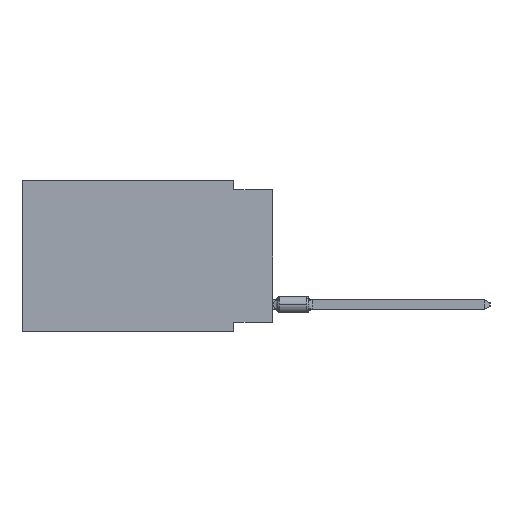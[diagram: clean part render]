
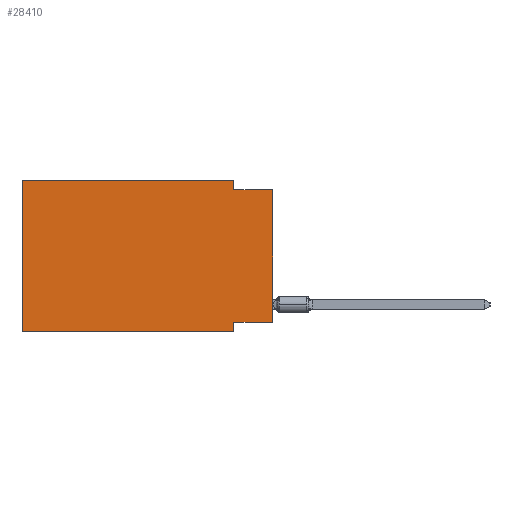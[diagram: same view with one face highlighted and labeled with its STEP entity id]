
A CAD part, left-side view. The second image highlights one B-rep face of the part: STEP entity #28410.
In plain terms, the highlighted planar face has unit normal (-1, 0, 0).
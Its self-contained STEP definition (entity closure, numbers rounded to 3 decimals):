
#1242 = DIRECTION ( 'NONE',  ( 0., 0., -1. ) ) ;
#1474 = CARTESIAN_POINT ( 'NONE',  ( 0., 0., -9.271 ) ) ;
#2126 = PLANE ( 'NONE',  #21336 ) ;
#3246 = VERTEX_POINT ( 'NONE', #35363 ) ;
#3310 = VERTEX_POINT ( 'NONE', #5053 ) ;
#4761 = CARTESIAN_POINT ( 'NONE',  ( 0., 2.54, -0.635 ) ) ;
#5053 = CARTESIAN_POINT ( 'NONE',  ( 0., 2.54, -9.906 ) ) ;
#6661 = ORIENTED_EDGE ( 'NONE', *, *, #19659, .F. ) ;
#7812 = VECTOR ( 'NONE', #42148, 1000. ) ;
#8633 = LINE ( 'NONE', #20342, #9895 ) ;
#8875 = CARTESIAN_POINT ( 'NONE',  ( 0., 16.383, 0. ) ) ;
#9584 = DIRECTION ( 'NONE',  ( 1., 0., 0. ) ) ;
#9895 = VECTOR ( 'NONE', #32807, 1000. ) ;
#10799 = CARTESIAN_POINT ( 'NONE',  ( 0., 0., 0. ) ) ;
#10932 = VECTOR ( 'NONE', #20970, 1000. ) ;
#11849 = DIRECTION ( 'NONE',  ( 0., -1., 0. ) ) ;
#11919 = CARTESIAN_POINT ( 'NONE',  ( 0., 16.383, 0. ) ) ;
#14776 = VERTEX_POINT ( 'NONE', #19033 ) ;
#14794 = LINE ( 'NONE', #25578, #43754 ) ;
#15599 = LINE ( 'NONE', #31794, #17666 ) ;
#17247 = VERTEX_POINT ( 'NONE', #35749 ) ;
#17666 = VECTOR ( 'NONE', #11849, 1000. ) ;
#18080 = VERTEX_POINT ( 'NONE', #1474 ) ;
#19033 = CARTESIAN_POINT ( 'NONE',  ( 0., 2.54, -9.271 ) ) ;
#19659 = EDGE_CURVE ( 'NONE', #27458, #28645, #37149, .T. ) ;
#20342 = CARTESIAN_POINT ( 'NONE',  ( 0., 0., -0.635 ) ) ;
#20970 = DIRECTION ( 'NONE',  ( 0., 0., -1. ) ) ;
#21336 = AXIS2_PLACEMENT_3D ( 'NONE', #26052, #9584, #50982 ) ;
#21464 = CARTESIAN_POINT ( 'NONE',  ( 0., 2.54, -9.906 ) ) ;
#24674 = CARTESIAN_POINT ( 'NONE',  ( 0., 2.54, 0. ) ) ;
#25031 = ORIENTED_EDGE ( 'NONE', *, *, #38498, .F. ) ;
#25089 = DIRECTION ( 'NONE',  ( 0., 0., 1. ) ) ;
#25493 = CARTESIAN_POINT ( 'NONE',  ( 0., 16.383, 0. ) ) ;
#25578 = CARTESIAN_POINT ( 'NONE',  ( 0., 0., -9.271 ) ) ;
#26052 = CARTESIAN_POINT ( 'NONE',  ( 0., 16.383, 0. ) ) ;
#26352 = ORIENTED_EDGE ( 'NONE', *, *, #51759, .F. ) ;
#27458 = VERTEX_POINT ( 'NONE', #24674 ) ;
#27761 = ORIENTED_EDGE ( 'NONE', *, *, #35617, .T. ) ;
#28410 = ADVANCED_FACE ( 'NONE', ( #45964 ), #2126, .F. ) ;
#28645 = VERTEX_POINT ( 'NONE', #4761 ) ;
#29615 = VECTOR ( 'NONE', #1242, 1000. ) ;
#30886 = EDGE_LOOP ( 'NONE', ( #27761, #42951, #6661, #26352, #36072, #34089, #25031, #50309 ) ) ;
#31596 = LINE ( 'NONE', #11919, #44057 ) ;
#31794 = CARTESIAN_POINT ( 'NONE',  ( 0., 16.383, -9.906 ) ) ;
#32807 = DIRECTION ( 'NONE',  ( 0., -1., 0. ) ) ;
#33303 = LINE ( 'NONE', #8875, #44378 ) ;
#34089 = ORIENTED_EDGE ( 'NONE', *, *, #38778, .T. ) ;
#35363 = CARTESIAN_POINT ( 'NONE',  ( 0., 16.383, -9.906 ) ) ;
#35617 = EDGE_CURVE ( 'NONE', #18080, #17247, #46134, .T. ) ;
#35749 = CARTESIAN_POINT ( 'NONE',  ( 0., 0., -0.635 ) ) ;
#36072 = ORIENTED_EDGE ( 'NONE', *, *, #46811, .F. ) ;
#36891 = VERTEX_POINT ( 'NONE', #25493 ) ;
#37115 = LINE ( 'NONE', #21464, #29615 ) ;
#37149 = LINE ( 'NONE', #45116, #10932 ) ;
#37567 = EDGE_CURVE ( 'NONE', #28645, #17247, #8633, .T. ) ;
#38498 = EDGE_CURVE ( 'NONE', #14776, #3310, #37115, .T. ) ;
#38778 = EDGE_CURVE ( 'NONE', #3246, #3310, #15599, .T. ) ;
#41759 = DIRECTION ( 'NONE',  ( 0., 1., 0. ) ) ;
#42148 = DIRECTION ( 'NONE',  ( 0., 0., 1. ) ) ;
#42951 = ORIENTED_EDGE ( 'NONE', *, *, #37567, .F. ) ;
#43754 = VECTOR ( 'NONE', #41759, 1000. ) ;
#44057 = VECTOR ( 'NONE', #44311, 1000. ) ;
#44311 = DIRECTION ( 'NONE',  ( 0., -1., 0. ) ) ;
#44378 = VECTOR ( 'NONE', #25089, 1000. ) ;
#45116 = CARTESIAN_POINT ( 'NONE',  ( 0., 2.54, 0. ) ) ;
#45964 = FACE_OUTER_BOUND ( 'NONE', #30886, .T. ) ;
#46134 = LINE ( 'NONE', #10799, #7812 ) ;
#46811 = EDGE_CURVE ( 'NONE', #3246, #36891, #33303, .T. ) ;
#49497 = EDGE_CURVE ( 'NONE', #18080, #14776, #14794, .T. ) ;
#50309 = ORIENTED_EDGE ( 'NONE', *, *, #49497, .F. ) ;
#50982 = DIRECTION ( 'NONE',  ( 0., 0., -1. ) ) ;
#51759 = EDGE_CURVE ( 'NONE', #36891, #27458, #31596, .T. ) ;
